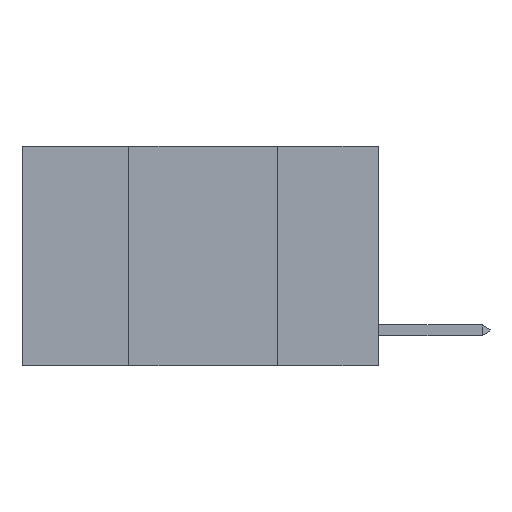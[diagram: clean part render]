
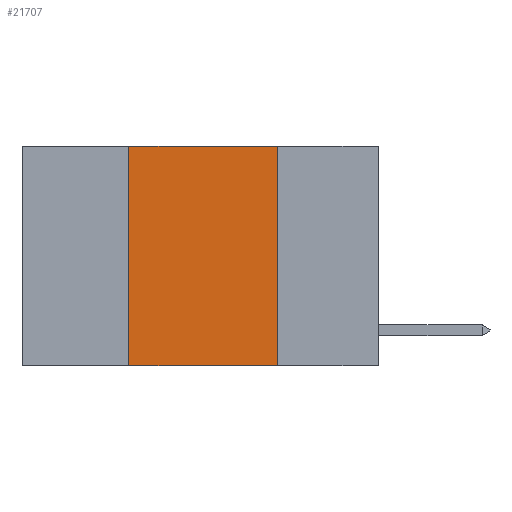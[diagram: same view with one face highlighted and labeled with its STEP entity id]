
A CAD part, left-side view. The second image highlights one B-rep face of the part: STEP entity #21707.
In plain terms, the highlighted planar face has unit normal (-1, 0, 0).
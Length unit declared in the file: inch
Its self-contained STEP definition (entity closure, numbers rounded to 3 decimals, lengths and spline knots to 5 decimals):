
#312 = CARTESIAN_POINT ( 'NONE',  ( 0., 0.6, 0. ) ) ;
#655 = EDGE_CURVE ( 'NONE', #8967, #2681, #9920, .T. ) ;
#1414 = ORIENTED_EDGE ( 'NONE', *, *, #8551, .T. ) ;
#1811 = FACE_OUTER_BOUND ( 'NONE', #7065, .T. ) ;
#1896 = DIRECTION ( 'NONE',  ( 0., 0., -1. ) ) ;
#2060 = VECTOR ( 'NONE', #26373, 39.37008 ) ;
#2165 = PLANE ( 'NONE',  #4760 ) ;
#2681 = VERTEX_POINT ( 'NONE', #26424 ) ;
#3251 = CARTESIAN_POINT ( 'NONE',  ( 0., 0.42, 0. ) ) ;
#4760 = AXIS2_PLACEMENT_3D ( 'NONE', #15369, #13346, #26558 ) ;
#7065 = EDGE_LOOP ( 'NONE', ( #23348, #9140, #8734, #1414 ) ) ;
#8551 = EDGE_CURVE ( 'NONE', #24660, #22807, #21185, .T. ) ;
#8734 = ORIENTED_EDGE ( 'NONE', *, *, #28120, .F. ) ;
#8967 = VERTEX_POINT ( 'NONE', #3251 ) ;
#9140 = ORIENTED_EDGE ( 'NONE', *, *, #655, .F. ) ;
#9920 = LINE ( 'NONE', #312, #21726 ) ;
#10221 = VECTOR ( 'NONE', #20782, 39.37008 ) ;
#11921 = CARTESIAN_POINT ( 'NONE',  ( 0., 0.42, 0. ) ) ;
#12147 = EDGE_CURVE ( 'NONE', #2681, #22807, #15636, .T. ) ;
#12956 = CARTESIAN_POINT ( 'NONE',  ( 0., 0.17, 0. ) ) ;
#13346 = DIRECTION ( 'NONE',  ( 1., 0., 0. ) ) ;
#15279 = CARTESIAN_POINT ( 'NONE',  ( 0., 0.6, -0.37 ) ) ;
#15369 = CARTESIAN_POINT ( 'NONE',  ( 0., 0.6, 0. ) ) ;
#15636 = LINE ( 'NONE', #12956, #26060 ) ;
#19549 = CARTESIAN_POINT ( 'NONE',  ( 0., 0.17, -0.37 ) ) ;
#20782 = DIRECTION ( 'NONE',  ( 0., 0., 1. ) ) ;
#21185 = LINE ( 'NONE', #15279, #2060 ) ;
#21222 = CARTESIAN_POINT ( 'NONE',  ( 0., 0.42, -0.37 ) ) ;
#21707 = ADVANCED_FACE ( 'NONE', ( #1811 ), #2165, .F. ) ;
#21726 = VECTOR ( 'NONE', #26801, 39.37008 ) ;
#22807 = VERTEX_POINT ( 'NONE', #19549 ) ;
#23348 = ORIENTED_EDGE ( 'NONE', *, *, #12147, .F. ) ;
#24660 = VERTEX_POINT ( 'NONE', #21222 ) ;
#25147 = LINE ( 'NONE', #11921, #10221 ) ;
#26060 = VECTOR ( 'NONE', #1896, 39.37008 ) ;
#26373 = DIRECTION ( 'NONE',  ( 0., -1., 0. ) ) ;
#26424 = CARTESIAN_POINT ( 'NONE',  ( 0., 0.17, 0. ) ) ;
#26558 = DIRECTION ( 'NONE',  ( 0., 0., -1. ) ) ;
#26801 = DIRECTION ( 'NONE',  ( 0., -1., 0. ) ) ;
#28120 = EDGE_CURVE ( 'NONE', #24660, #8967, #25147, .T. ) ;
